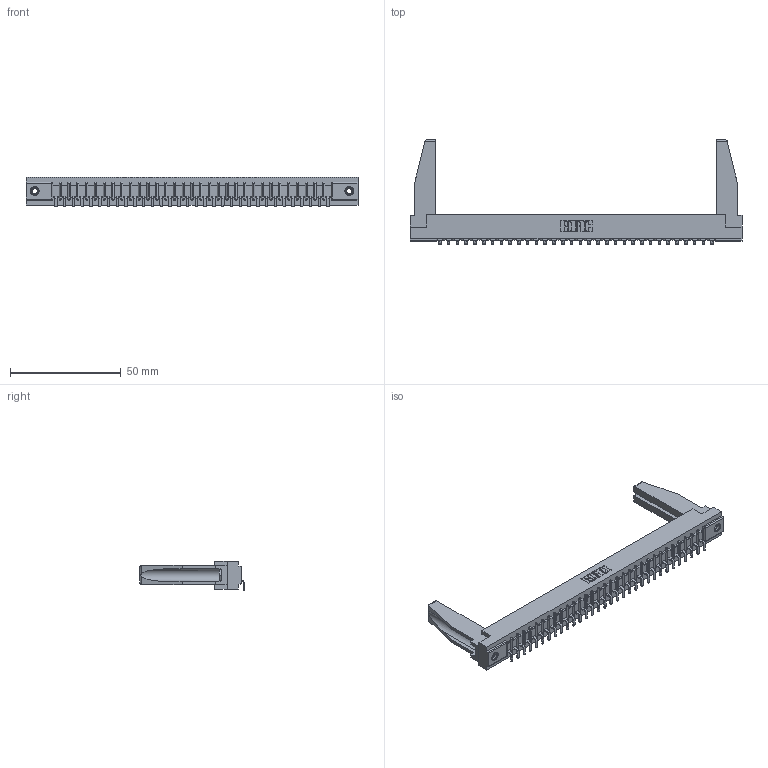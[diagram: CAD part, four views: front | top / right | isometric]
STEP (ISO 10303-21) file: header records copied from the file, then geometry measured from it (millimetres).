
FILE_DESCRIPTION (( 'STEP AP203' ), '1' );
FILE_NAME ('357-032-453-178.STEP', '2020-10-02T06:13:19', ( '' ), ( '' ), 'SwSTEP 2.0', 'SolidWorks 2020', '' );
FILE_SCHEMA (( 'CONFIG_CONTROL_DESIGN' ));
Length unit declared in the file: inch
Products named in the file (5): 345-250-001_345-250-001-102; 307-220-078; 307 Part_.156 Dia Mounting Holes; 307-290-002_553; 357-032-453-178
Assembly tree (37 placements, depth 2):
  357-032-453-178
    307 Part_.156 Dia Mounting Holes
    307-290-002_553  x32
    307-220-078  x2
    345-250-001_345-250-001-102  x2
Bounding box: 149.81 x 47.03 x 13.5 mm (x, y, z)
Volume: 19950.1 mm3; surface area: 23664.5 mm2
Topology: 37 solids, 37 shells, 2777 faces, 8461 edges, 5542 vertices
Faces by surface type: plane 1658, cylinder 1037, sphere 66, cone 12, torus 4
Entity records: 31959 total; most frequent: CARTESIAN_POINT 5390, ORIENTED_EDGE 5336, DIRECTION 5198, EDGE_CURVE 2668, VECTOR 2042, LINE 2042, VERTEX_POINT 1728, AXIS2_PLACEMENT_3D 1578
